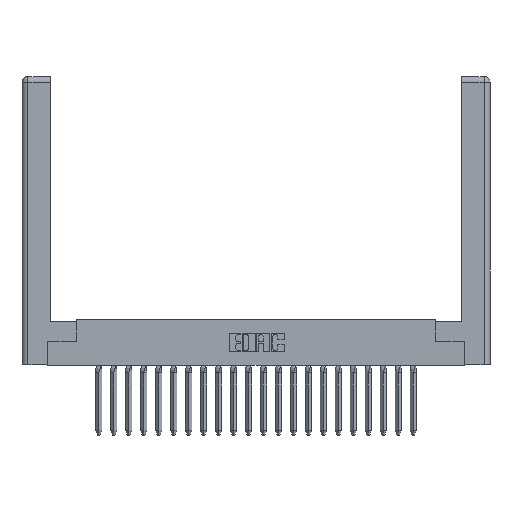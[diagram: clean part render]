
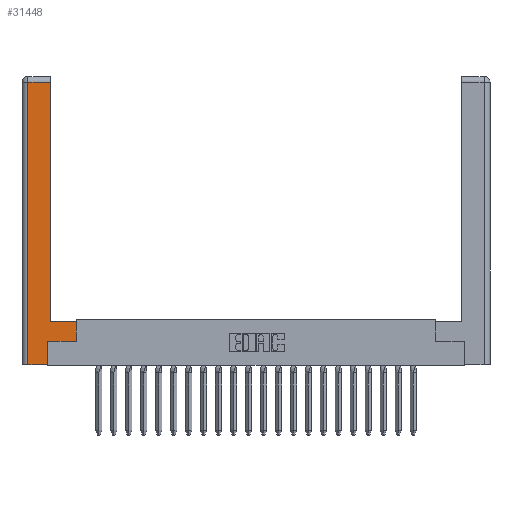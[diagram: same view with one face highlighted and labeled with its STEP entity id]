
A CAD part, top view. The second image highlights one B-rep face of the part: STEP entity #31448.
In plain terms, the highlighted planar face has unit normal (0, 0, 1).
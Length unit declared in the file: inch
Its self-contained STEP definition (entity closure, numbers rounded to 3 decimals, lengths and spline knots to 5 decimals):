
#291 = CARTESIAN_POINT ( 'NONE',  ( 0.0615, 0., 0. ) ) ;
#487 = VERTEX_POINT ( 'NONE', #39776 ) ;
#1089 = EDGE_CURVE ( 'NONE', #43758, #487, #16950, .T. ) ;
#4160 = LINE ( 'NONE', #42760, #28861 ) ;
#4698 = CARTESIAN_POINT ( 'NONE',  ( 0.295, 2.94, 0. ) ) ;
#5321 = ORIENTED_EDGE ( 'NONE', *, *, #1089, .T. ) ;
#5824 = CARTESIAN_POINT ( 'NONE',  ( 0.0615, 0., 0. ) ) ;
#6016 = VECTOR ( 'NONE', #44007, 39.37008 ) ;
#6699 = LINE ( 'NONE', #291, #45738 ) ;
#6917 = CARTESIAN_POINT ( 'NONE',  ( 0.265, 0., 0. ) ) ;
#7689 = DIRECTION ( 'NONE',  ( 0., 0., -1. ) ) ;
#8781 = EDGE_LOOP ( 'NONE', ( #40612, #30796, #21939, #5321, #37910, #32800, #22620, #12322 ) ) ;
#8936 = CARTESIAN_POINT ( 'NONE',  ( 0.0615, 2.94, 0. ) ) ;
#9657 = LINE ( 'NONE', #34226, #22908 ) ;
#10624 = DIRECTION ( 'NONE',  ( 1., 0., 0. ) ) ;
#10692 = EDGE_CURVE ( 'NONE', #27830, #16990, #45136, .T. ) ;
#10959 = CARTESIAN_POINT ( 'NONE',  ( 0.565, 0.245, 0. ) ) ;
#12322 = ORIENTED_EDGE ( 'NONE', *, *, #23696, .T. ) ;
#12804 = EDGE_CURVE ( 'NONE', #39047, #23307, #9657, .T. ) ;
#14499 = FACE_OUTER_BOUND ( 'NONE', #8781, .T. ) ;
#15745 = EDGE_CURVE ( 'NONE', #16990, #25132, #38640, .T. ) ;
#16720 = AXIS2_PLACEMENT_3D ( 'NONE', #29673, #7689, #33387 ) ;
#16950 = LINE ( 'NONE', #6917, #46184 ) ;
#16990 = VERTEX_POINT ( 'NONE', #4698 ) ;
#19610 = DIRECTION ( 'NONE',  ( 1., 0., 0. ) ) ;
#19817 = LINE ( 'NONE', #40341, #6016 ) ;
#19838 = CARTESIAN_POINT ( 'NONE',  ( 0.295, 0.45, 0. ) ) ;
#20630 = VECTOR ( 'NONE', #40117, 39.37008 ) ;
#21939 = ORIENTED_EDGE ( 'NONE', *, *, #37475, .T. ) ;
#22620 = ORIENTED_EDGE ( 'NONE', *, *, #43967, .T. ) ;
#22908 = VECTOR ( 'NONE', #19610, 39.37008 ) ;
#23307 = VERTEX_POINT ( 'NONE', #10959 ) ;
#23696 = EDGE_CURVE ( 'NONE', #24270, #27830, #33865, .T. ) ;
#24270 = VERTEX_POINT ( 'NONE', #24286 ) ;
#24286 = CARTESIAN_POINT ( 'NONE',  ( 0.565, 0.45, 0. ) ) ;
#24417 = CARTESIAN_POINT ( 'NONE',  ( 0.265, 0.245, 0. ) ) ;
#25121 = CARTESIAN_POINT ( 'NONE',  ( 0.0615, 2.94, 0. ) ) ;
#25132 = VERTEX_POINT ( 'NONE', #25121 ) ;
#26059 = DIRECTION ( 'NONE',  ( 0., 1., 0. ) ) ;
#27096 = DIRECTION ( 'NONE',  ( -1., 0., 0. ) ) ;
#27830 = VERTEX_POINT ( 'NONE', #19838 ) ;
#27975 = DIRECTION ( 'NONE',  ( 0., 1., 0. ) ) ;
#28861 = VECTOR ( 'NONE', #27975, 39.37008 ) ;
#29673 = CARTESIAN_POINT ( 'NONE',  ( 0., 0., 0. ) ) ;
#29698 = DIRECTION ( 'NONE',  ( 0., -1., 0. ) ) ;
#30796 = ORIENTED_EDGE ( 'NONE', *, *, #15745, .T. ) ;
#31448 = ADVANCED_FACE ( 'NONE', ( #14499 ), #44258, .F. ) ;
#32800 = ORIENTED_EDGE ( 'NONE', *, *, #12804, .T. ) ;
#32886 = VECTOR ( 'NONE', #27096, 39.37008 ) ;
#33387 = DIRECTION ( 'NONE',  ( -1., 0., 0. ) ) ;
#33732 = VECTOR ( 'NONE', #26059, 39.37008 ) ;
#33865 = LINE ( 'NONE', #36602, #20630 ) ;
#34226 = CARTESIAN_POINT ( 'NONE',  ( 0.565, 0.245, 0. ) ) ;
#36602 = CARTESIAN_POINT ( 'NONE',  ( 0.295, 0.45, 0. ) ) ;
#37475 = EDGE_CURVE ( 'NONE', #25132, #43758, #6699, .T. ) ;
#37910 = ORIENTED_EDGE ( 'NONE', *, *, #45601, .T. ) ;
#38640 = LINE ( 'NONE', #8936, #32886 ) ;
#39047 = VERTEX_POINT ( 'NONE', #24417 ) ;
#39776 = CARTESIAN_POINT ( 'NONE',  ( 0.265, 0., 0. ) ) ;
#40117 = DIRECTION ( 'NONE',  ( -1., 0., 0. ) ) ;
#40341 = CARTESIAN_POINT ( 'NONE',  ( 0.565, 0.45, 0. ) ) ;
#40612 = ORIENTED_EDGE ( 'NONE', *, *, #10692, .T. ) ;
#42760 = CARTESIAN_POINT ( 'NONE',  ( 0.265, 0.245, 0. ) ) ;
#43758 = VERTEX_POINT ( 'NONE', #5824 ) ;
#43967 = EDGE_CURVE ( 'NONE', #23307, #24270, #19817, .T. ) ;
#44007 = DIRECTION ( 'NONE',  ( 0., 1., 0. ) ) ;
#44258 = PLANE ( 'NONE',  #16720 ) ;
#44487 = CARTESIAN_POINT ( 'NONE',  ( 0.295, 3., 0. ) ) ;
#45136 = LINE ( 'NONE', #44487, #33732 ) ;
#45601 = EDGE_CURVE ( 'NONE', #487, #39047, #4160, .T. ) ;
#45738 = VECTOR ( 'NONE', #29698, 39.37008 ) ;
#46184 = VECTOR ( 'NONE', #10624, 39.37008 ) ;
